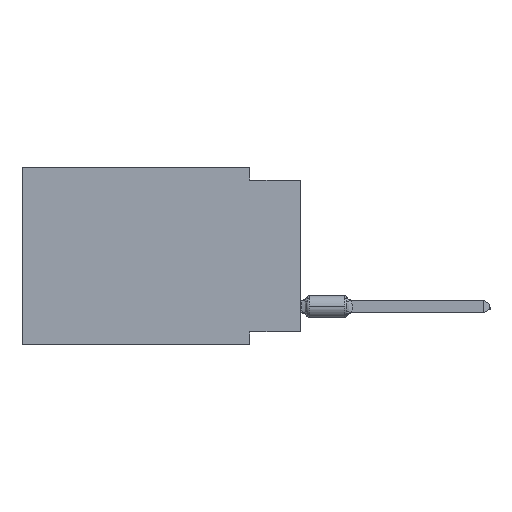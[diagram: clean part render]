
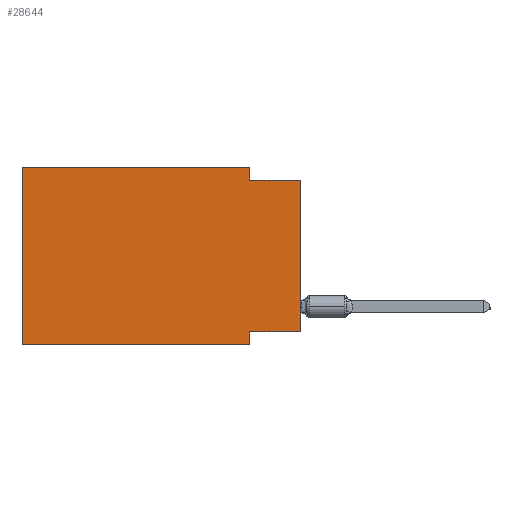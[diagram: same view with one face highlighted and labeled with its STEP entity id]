
A CAD part, left-side view. The second image highlights one B-rep face of the part: STEP entity #28644.
In plain terms, the highlighted planar face has unit normal (-1, 0, 0).
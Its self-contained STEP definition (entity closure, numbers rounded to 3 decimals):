
#850 = PLANE ( 'NONE',  #7136 ) ;
#1037 = CARTESIAN_POINT ( 'NONE',  ( 0., 13.97, 0. ) ) ;
#1434 = CARTESIAN_POINT ( 'NONE',  ( 0., 2.54, 0. ) ) ;
#1747 = CARTESIAN_POINT ( 'NONE',  ( 0., 0., -8.255 ) ) ;
#1888 = CARTESIAN_POINT ( 'NONE',  ( 0., 13.97, -8.89 ) ) ;
#2892 = CARTESIAN_POINT ( 'NONE',  ( 0., 13.97, 0. ) ) ;
#4746 = CARTESIAN_POINT ( 'NONE',  ( 0., 0., -0.635 ) ) ;
#5603 = VERTEX_POINT ( 'NONE', #20944 ) ;
#6031 = EDGE_LOOP ( 'NONE', ( #21230, #22054, #17142, #44802, #11818, #19062, #42150, #30986 ) ) ;
#6656 = VECTOR ( 'NONE', #37657, 1000. ) ;
#7136 = AXIS2_PLACEMENT_3D ( 'NONE', #25591, #8773, #21621 ) ;
#7528 = CARTESIAN_POINT ( 'NONE',  ( 0., 2.54, 0. ) ) ;
#7614 = EDGE_CURVE ( 'NONE', #48225, #37501, #14341, .T. ) ;
#8099 = EDGE_CURVE ( 'NONE', #5603, #21047, #31861, .T. ) ;
#8655 = VECTOR ( 'NONE', #34039, 1000. ) ;
#8773 = DIRECTION ( 'NONE',  ( 1., 0., 0. ) ) ;
#10406 = CARTESIAN_POINT ( 'NONE',  ( 0., 2.54, -8.89 ) ) ;
#10767 = VECTOR ( 'NONE', #26433, 1000. ) ;
#11818 = ORIENTED_EDGE ( 'NONE', *, *, #17234, .F. ) ;
#11848 = DIRECTION ( 'NONE',  ( 0., -1., 0. ) ) ;
#13139 = CARTESIAN_POINT ( 'NONE',  ( 0., 0., 0. ) ) ;
#14341 = LINE ( 'NONE', #10406, #10767 ) ;
#17142 = ORIENTED_EDGE ( 'NONE', *, *, #17400, .F. ) ;
#17234 = EDGE_CURVE ( 'NONE', #17409, #37140, #21561, .T. ) ;
#17400 = EDGE_CURVE ( 'NONE', #32258, #5603, #25124, .T. ) ;
#17409 = VERTEX_POINT ( 'NONE', #49636 ) ;
#19045 = CARTESIAN_POINT ( 'NONE',  ( 0., 0., -8.255 ) ) ;
#19062 = ORIENTED_EDGE ( 'NONE', *, *, #21270, .T. ) ;
#19469 = CARTESIAN_POINT ( 'NONE',  ( 0., 0., -0.635 ) ) ;
#19709 = EDGE_CURVE ( 'NONE', #28376, #21047, #28946, .T. ) ;
#20944 = CARTESIAN_POINT ( 'NONE',  ( 0., 2.54, -0.635 ) ) ;
#21047 = VERTEX_POINT ( 'NONE', #4746 ) ;
#21230 = ORIENTED_EDGE ( 'NONE', *, *, #19709, .T. ) ;
#21270 = EDGE_CURVE ( 'NONE', #17409, #37501, #26093, .T. ) ;
#21561 = LINE ( 'NONE', #1037, #6656 ) ;
#21621 = DIRECTION ( 'NONE',  ( 0., 0., -1. ) ) ;
#21719 = CARTESIAN_POINT ( 'NONE',  ( 0., 13.97, 0. ) ) ;
#22054 = ORIENTED_EDGE ( 'NONE', *, *, #8099, .F. ) ;
#22612 = VECTOR ( 'NONE', #11848, 1000. ) ;
#23596 = CARTESIAN_POINT ( 'NONE',  ( 0., 2.54, -8.255 ) ) ;
#25124 = LINE ( 'NONE', #1434, #32784 ) ;
#25591 = CARTESIAN_POINT ( 'NONE',  ( 0., 13.97, 0. ) ) ;
#25948 = LINE ( 'NONE', #1747, #35742 ) ;
#26093 = LINE ( 'NONE', #1888, #8655 ) ;
#26433 = DIRECTION ( 'NONE',  ( 0., 0., -1. ) ) ;
#28376 = VERTEX_POINT ( 'NONE', #19045 ) ;
#28644 = ADVANCED_FACE ( 'NONE', ( #28770 ), #850, .F. ) ;
#28770 = FACE_OUTER_BOUND ( 'NONE', #6031, .T. ) ;
#28946 = LINE ( 'NONE', #13139, #49899 ) ;
#29188 = CARTESIAN_POINT ( 'NONE',  ( 0., 2.54, -8.89 ) ) ;
#30986 = ORIENTED_EDGE ( 'NONE', *, *, #50720, .F. ) ;
#31861 = LINE ( 'NONE', #19469, #22612 ) ;
#32258 = VERTEX_POINT ( 'NONE', #7528 ) ;
#32784 = VECTOR ( 'NONE', #45434, 1000. ) ;
#34039 = DIRECTION ( 'NONE',  ( 0., -1., 0. ) ) ;
#35742 = VECTOR ( 'NONE', #37570, 1000. ) ;
#36594 = DIRECTION ( 'NONE',  ( 0., 0., 1. ) ) ;
#37140 = VERTEX_POINT ( 'NONE', #2892 ) ;
#37501 = VERTEX_POINT ( 'NONE', #29188 ) ;
#37556 = DIRECTION ( 'NONE',  ( 0., -1., 0. ) ) ;
#37570 = DIRECTION ( 'NONE',  ( 0., 1., 0. ) ) ;
#37657 = DIRECTION ( 'NONE',  ( 0., 0., 1. ) ) ;
#39673 = VECTOR ( 'NONE', #37556, 1000. ) ;
#42150 = ORIENTED_EDGE ( 'NONE', *, *, #7614, .F. ) ;
#44802 = ORIENTED_EDGE ( 'NONE', *, *, #48370, .F. ) ;
#45434 = DIRECTION ( 'NONE',  ( 0., 0., -1. ) ) ;
#45476 = LINE ( 'NONE', #21719, #39673 ) ;
#48225 = VERTEX_POINT ( 'NONE', #23596 ) ;
#48370 = EDGE_CURVE ( 'NONE', #37140, #32258, #45476, .T. ) ;
#49636 = CARTESIAN_POINT ( 'NONE',  ( 0., 13.97, -8.89 ) ) ;
#49899 = VECTOR ( 'NONE', #36594, 1000. ) ;
#50720 = EDGE_CURVE ( 'NONE', #28376, #48225, #25948, .T. ) ;
